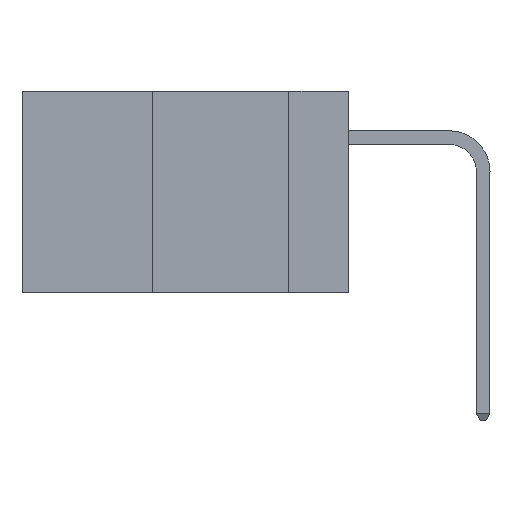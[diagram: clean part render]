
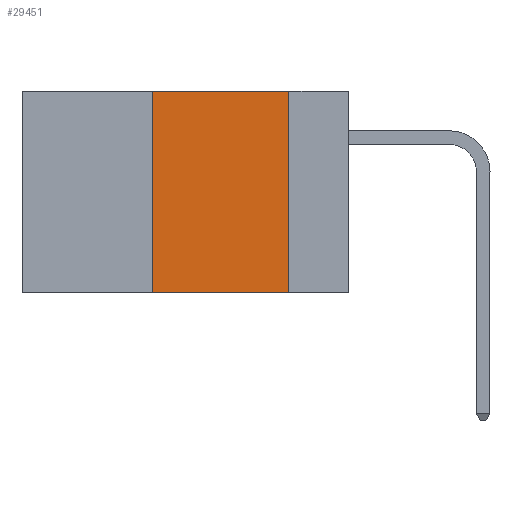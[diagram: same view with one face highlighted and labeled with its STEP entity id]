
A CAD part, left-side view. The second image highlights one B-rep face of the part: STEP entity #29451.
In plain terms, the highlighted planar face has unit normal (-1, 0, 0).
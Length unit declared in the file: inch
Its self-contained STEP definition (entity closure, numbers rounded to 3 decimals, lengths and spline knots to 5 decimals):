
#373 = EDGE_CURVE ( 'NONE', #11688, #26219, #24664, .T. ) ;
#2414 = DIRECTION ( 'NONE',  ( 0., -1., 0. ) ) ;
#2577 = VERTEX_POINT ( 'NONE', #16447 ) ;
#5074 = DIRECTION ( 'NONE',  ( 0., 0., -1. ) ) ;
#5251 = LINE ( 'NONE', #17842, #29858 ) ;
#5366 = CARTESIAN_POINT ( 'NONE',  ( 0., 0.11, 0. ) ) ;
#6101 = EDGE_CURVE ( 'NONE', #22512, #26219, #5251, .T. ) ;
#6138 = ORIENTED_EDGE ( 'NONE', *, *, #11340, .F. ) ;
#7088 = VECTOR ( 'NONE', #2414, 39.37008 ) ;
#7387 = CARTESIAN_POINT ( 'NONE',  ( 0., 0.6, 0. ) ) ;
#8228 = FACE_OUTER_BOUND ( 'NONE', #21103, .T. ) ;
#10800 = DIRECTION ( 'NONE',  ( 0., -1., 0. ) ) ;
#11340 = EDGE_CURVE ( 'NONE', #2577, #11688, #20129, .T. ) ;
#11599 = VECTOR ( 'NONE', #29466, 39.37008 ) ;
#11688 = VERTEX_POINT ( 'NONE', #16761 ) ;
#11724 = CARTESIAN_POINT ( 'NONE',  ( 0., 0.11, -0.37 ) ) ;
#12334 = ORIENTED_EDGE ( 'NONE', *, *, #6101, .T. ) ;
#12720 = VECTOR ( 'NONE', #24173, 39.37008 ) ;
#14535 = EDGE_CURVE ( 'NONE', #22512, #2577, #31480, .T. ) ;
#14858 = PLANE ( 'NONE',  #22969 ) ;
#16447 = CARTESIAN_POINT ( 'NONE',  ( 0., 0.36, 0. ) ) ;
#16761 = CARTESIAN_POINT ( 'NONE',  ( 0., 0.11, 0. ) ) ;
#17325 = CARTESIAN_POINT ( 'NONE',  ( 0., 0.6, 0. ) ) ;
#17842 = CARTESIAN_POINT ( 'NONE',  ( 0., 0.6, -0.37 ) ) ;
#19199 = CARTESIAN_POINT ( 'NONE',  ( 0., 0.36, 0. ) ) ;
#19774 = DIRECTION ( 'NONE',  ( 1., 0., 0. ) ) ;
#20129 = LINE ( 'NONE', #7387, #7088 ) ;
#21103 = EDGE_LOOP ( 'NONE', ( #31266, #6138, #24161, #12334 ) ) ;
#21961 = CARTESIAN_POINT ( 'NONE',  ( 0., 0.36, -0.37 ) ) ;
#22512 = VERTEX_POINT ( 'NONE', #21961 ) ;
#22969 = AXIS2_PLACEMENT_3D ( 'NONE', #17325, #19774, #5074 ) ;
#24161 = ORIENTED_EDGE ( 'NONE', *, *, #14535, .F. ) ;
#24173 = DIRECTION ( 'NONE',  ( 0., 0., 1. ) ) ;
#24664 = LINE ( 'NONE', #5366, #11599 ) ;
#26219 = VERTEX_POINT ( 'NONE', #11724 ) ;
#29451 = ADVANCED_FACE ( 'NONE', ( #8228 ), #14858, .F. ) ;
#29466 = DIRECTION ( 'NONE',  ( 0., 0., -1. ) ) ;
#29858 = VECTOR ( 'NONE', #10800, 39.37008 ) ;
#31266 = ORIENTED_EDGE ( 'NONE', *, *, #373, .F. ) ;
#31480 = LINE ( 'NONE', #19199, #12720 ) ;
